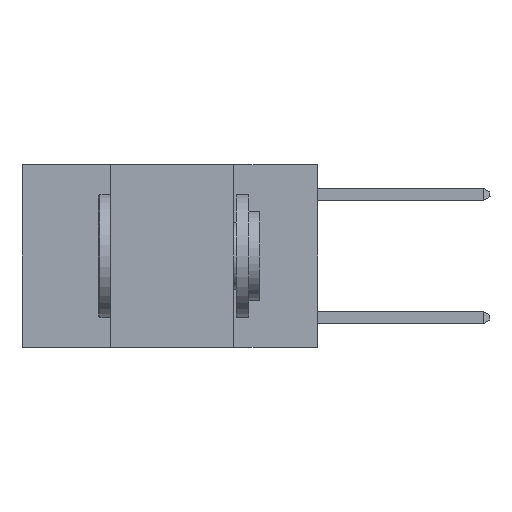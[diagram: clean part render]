
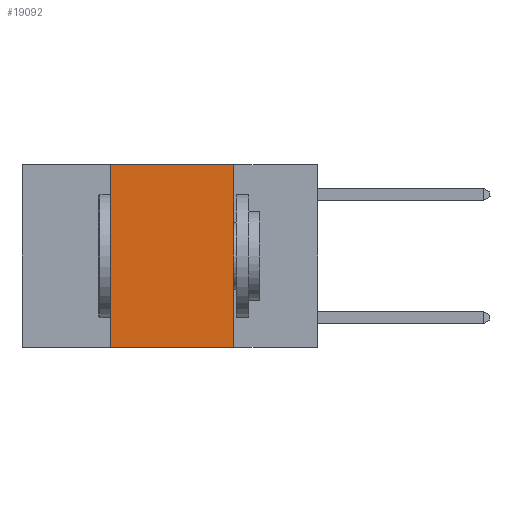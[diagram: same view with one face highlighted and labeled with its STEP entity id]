
A CAD part, left-side view. The second image highlights one B-rep face of the part: STEP entity #19092.
In plain terms, the highlighted planar face has unit normal (-1, 0, 0).
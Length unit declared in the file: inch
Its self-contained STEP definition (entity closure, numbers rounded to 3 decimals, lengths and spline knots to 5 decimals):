
#723 = FACE_OUTER_BOUND ( 'NONE', #18582, .T. ) ;
#884 = DIRECTION ( 'NONE',  ( 0., -1., 0. ) ) ;
#2053 = PLANE ( 'NONE',  #16541 ) ;
#2690 = CARTESIAN_POINT ( 'NONE',  ( 0., 0.17, -0.37 ) ) ;
#2831 = ORIENTED_EDGE ( 'NONE', *, *, #16884, .F. ) ;
#3542 = EDGE_CURVE ( 'NONE', #19330, #15289, #5460, .T. ) ;
#3910 = LINE ( 'NONE', #10473, #20314 ) ;
#3979 = DIRECTION ( 'NONE',  ( 0., 0., -1. ) ) ;
#4010 = VECTOR ( 'NONE', #4852, 39.37008 ) ;
#4852 = DIRECTION ( 'NONE',  ( 0., 0., 1. ) ) ;
#5401 = CARTESIAN_POINT ( 'NONE',  ( 0., 0.6, 0. ) ) ;
#5460 = LINE ( 'NONE', #12049, #10830 ) ;
#6773 = CARTESIAN_POINT ( 'NONE',  ( 0., 0.42, 0. ) ) ;
#6786 = VECTOR ( 'NONE', #14363, 39.37008 ) ;
#6792 = CARTESIAN_POINT ( 'NONE',  ( 0., 0.17, 0. ) ) ;
#8020 = CARTESIAN_POINT ( 'NONE',  ( 0., 0.42, -0.37 ) ) ;
#8868 = DIRECTION ( 'NONE',  ( 0., 0., -1. ) ) ;
#9220 = VERTEX_POINT ( 'NONE', #8020 ) ;
#9641 = EDGE_CURVE ( 'NONE', #9220, #19330, #10103, .T. ) ;
#10103 = LINE ( 'NONE', #6773, #4010 ) ;
#10473 = CARTESIAN_POINT ( 'NONE',  ( 0., 0.17, 0. ) ) ;
#10750 = ORIENTED_EDGE ( 'NONE', *, *, #3542, .F. ) ;
#10830 = VECTOR ( 'NONE', #884, 39.37008 ) ;
#11240 = ORIENTED_EDGE ( 'NONE', *, *, #15559, .T. ) ;
#12049 = CARTESIAN_POINT ( 'NONE',  ( 0., 0.6, 0. ) ) ;
#13296 = ORIENTED_EDGE ( 'NONE', *, *, #9641, .F. ) ;
#14363 = DIRECTION ( 'NONE',  ( 0., -1., 0. ) ) ;
#15289 = VERTEX_POINT ( 'NONE', #6792 ) ;
#15493 = VERTEX_POINT ( 'NONE', #2690 ) ;
#15559 = EDGE_CURVE ( 'NONE', #9220, #15493, #19651, .T. ) ;
#16306 = CARTESIAN_POINT ( 'NONE',  ( 0., 0.6, -0.37 ) ) ;
#16541 = AXIS2_PLACEMENT_3D ( 'NONE', #5401, #17306, #3979 ) ;
#16884 = EDGE_CURVE ( 'NONE', #15289, #15493, #3910, .T. ) ;
#17306 = DIRECTION ( 'NONE',  ( 1., 0., 0. ) ) ;
#18582 = EDGE_LOOP ( 'NONE', ( #2831, #10750, #13296, #11240 ) ) ;
#19031 = CARTESIAN_POINT ( 'NONE',  ( 0., 0.42, 0. ) ) ;
#19092 = ADVANCED_FACE ( 'NONE', ( #723 ), #2053, .F. ) ;
#19330 = VERTEX_POINT ( 'NONE', #19031 ) ;
#19651 = LINE ( 'NONE', #16306, #6786 ) ;
#20314 = VECTOR ( 'NONE', #8868, 39.37008 ) ;
